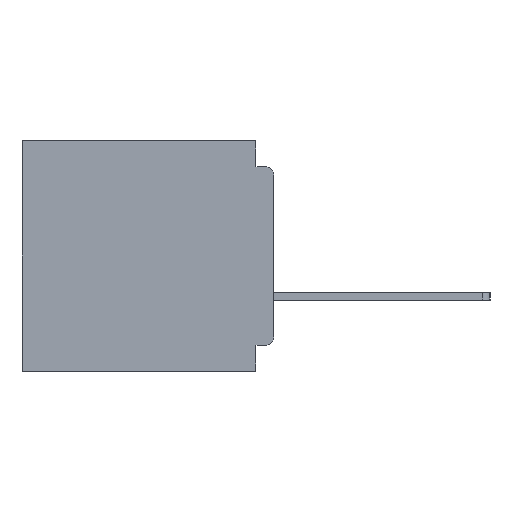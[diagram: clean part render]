
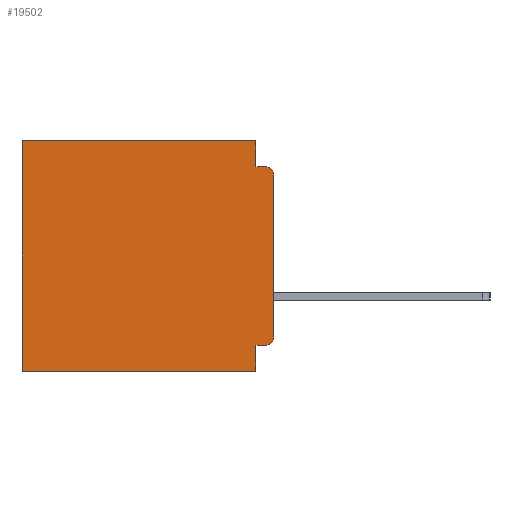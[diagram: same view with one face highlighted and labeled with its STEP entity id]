
A CAD part, left-side view. The second image highlights one B-rep face of the part: STEP entity #19502.
In plain terms, the highlighted planar face has unit normal (-1, 0, 0).
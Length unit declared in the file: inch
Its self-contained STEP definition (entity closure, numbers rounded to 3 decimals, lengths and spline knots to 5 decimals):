
#109 = CARTESIAN_POINT ( 'NONE',  ( 0.3, 0.015, -0.06 ) ) ;
#2106 = CARTESIAN_POINT ( 'NONE',  ( 0.3, 0.031, -0.4 ) ) ;
#2491 = EDGE_CURVE ( 'NONE', #35536, #6198, #42224, .T. ) ;
#3070 = LINE ( 'NONE', #46973, #23759 ) ;
#3792 = CIRCLE ( 'NONE', #16399, 0.015 ) ;
#3993 = CARTESIAN_POINT ( 'NONE',  ( 0.3, 0.437, -0.4 ) ) ;
#4067 = DIRECTION ( 'NONE',  ( 0., 0., -1. ) ) ;
#5150 = VECTOR ( 'NONE', #17080, 39.37008 ) ;
#5517 = CARTESIAN_POINT ( 'NONE',  ( 0.3, 0., -0.4 ) ) ;
#5836 = CARTESIAN_POINT ( 'NONE',  ( 0.3, 0.437, -0.4 ) ) ;
#6198 = VERTEX_POINT ( 'NONE', #5836 ) ;
#6887 = VERTEX_POINT ( 'NONE', #41497 ) ;
#7375 = VECTOR ( 'NONE', #49950, 39.37008 ) ;
#7682 = VECTOR ( 'NONE', #23790, 39.37008 ) ;
#9393 = ORIENTED_EDGE ( 'NONE', *, *, #21697, .F. ) ;
#9768 = ORIENTED_EDGE ( 'NONE', *, *, #14271, .F. ) ;
#10894 = VERTEX_POINT ( 'NONE', #34043 ) ;
#11126 = AXIS2_PLACEMENT_3D ( 'NONE', #14914, #41953, #18808 ) ;
#11199 = CARTESIAN_POINT ( 'NONE',  ( 0.3, 0.031, -0.355 ) ) ;
#11205 = CARTESIAN_POINT ( 'NONE',  ( 0.3, 0.031, 0. ) ) ;
#11536 = ORIENTED_EDGE ( 'NONE', *, *, #36013, .T. ) ;
#11788 = DIRECTION ( 'NONE',  ( 0., 0., -1. ) ) ;
#13599 = EDGE_CURVE ( 'NONE', #49246, #6198, #19241, .T. ) ;
#14271 = EDGE_CURVE ( 'NONE', #6887, #27284, #48869, .T. ) ;
#14914 = CARTESIAN_POINT ( 'NONE',  ( 0.3, 0.015, -0.34 ) ) ;
#15825 = CARTESIAN_POINT ( 'NONE',  ( 0.3, 0.031, -0.4 ) ) ;
#15903 = CARTESIAN_POINT ( 'NONE',  ( 0.3, 0.437, 0. ) ) ;
#16375 = DIRECTION ( 'NONE',  ( 1., 0., 0. ) ) ;
#16399 = AXIS2_PLACEMENT_3D ( 'NONE', #109, #27318, #4067 ) ;
#17080 = DIRECTION ( 'NONE',  ( 0., 0., -1. ) ) ;
#17122 = DIRECTION ( 'NONE',  ( 0., 1., 0. ) ) ;
#17203 = CARTESIAN_POINT ( 'NONE',  ( 0.3, 0.031, 0. ) ) ;
#18485 = FACE_OUTER_BOUND ( 'NONE', #36540, .T. ) ;
#18808 = DIRECTION ( 'NONE',  ( 0., 0., -1. ) ) ;
#18819 = ORIENTED_EDGE ( 'NONE', *, *, #21983, .T. ) ;
#19100 = EDGE_CURVE ( 'NONE', #24265, #35536, #31268, .T. ) ;
#19241 = LINE ( 'NONE', #3993, #38600 ) ;
#19502 = ADVANCED_FACE ( 'NONE', ( #18485 ), #31776, .F. ) ;
#19882 = CARTESIAN_POINT ( 'NONE',  ( 0.3, 0., -0.045 ) ) ;
#20841 = ORIENTED_EDGE ( 'NONE', *, *, #45400, .F. ) ;
#21107 = LINE ( 'NONE', #44178, #40495 ) ;
#21475 = DIRECTION ( 'NONE',  ( 0., 0., -1. ) ) ;
#21664 = VECTOR ( 'NONE', #45817, 39.37008 ) ;
#21697 = EDGE_CURVE ( 'NONE', #22167, #6887, #40722, .T. ) ;
#21983 = EDGE_CURVE ( 'NONE', #22167, #49246, #3070, .T. ) ;
#22167 = VERTEX_POINT ( 'NONE', #17203 ) ;
#23028 = EDGE_CURVE ( 'NONE', #31654, #27360, #27892, .T. ) ;
#23759 = VECTOR ( 'NONE', #31605, 39.37008 ) ;
#23790 = DIRECTION ( 'NONE',  ( 0., -1., 0. ) ) ;
#24265 = VERTEX_POINT ( 'NONE', #11199 ) ;
#25799 = CARTESIAN_POINT ( 'NONE',  ( 0.3, 0.015, -0.355 ) ) ;
#27284 = VERTEX_POINT ( 'NONE', #32142 ) ;
#27318 = DIRECTION ( 'NONE',  ( -1., 0., 0. ) ) ;
#27360 = VERTEX_POINT ( 'NONE', #36517 ) ;
#27892 = CIRCLE ( 'NONE', #11126, 0.015 ) ;
#27903 = CARTESIAN_POINT ( 'NONE',  ( 0.3, 0., -0.4 ) ) ;
#30729 = ORIENTED_EDGE ( 'NONE', *, *, #13599, .T. ) ;
#31268 = LINE ( 'NONE', #2106, #39122 ) ;
#31599 = ORIENTED_EDGE ( 'NONE', *, *, #2491, .F. ) ;
#31605 = DIRECTION ( 'NONE',  ( 0., 1., 0. ) ) ;
#31654 = VERTEX_POINT ( 'NONE', #25799 ) ;
#31776 = PLANE ( 'NONE',  #49595 ) ;
#32142 = CARTESIAN_POINT ( 'NONE',  ( 0.3, 0.015, -0.045 ) ) ;
#33873 = ORIENTED_EDGE ( 'NONE', *, *, #19100, .F. ) ;
#34043 = CARTESIAN_POINT ( 'NONE',  ( 0.3, 0., -0.06 ) ) ;
#34860 = ORIENTED_EDGE ( 'NONE', *, *, #43773, .F. ) ;
#35536 = VERTEX_POINT ( 'NONE', #15825 ) ;
#35546 = ORIENTED_EDGE ( 'NONE', *, *, #23028, .T. ) ;
#36013 = EDGE_CURVE ( 'NONE', #10894, #27284, #3792, .T. ) ;
#36517 = CARTESIAN_POINT ( 'NONE',  ( 0.3, 0., -0.34 ) ) ;
#36540 = EDGE_LOOP ( 'NONE', ( #20841, #11536, #9768, #9393, #18819, #30729, #31599, #33873, #34860, #35546 ) ) ;
#38600 = VECTOR ( 'NONE', #11788, 39.37008 ) ;
#39122 = VECTOR ( 'NONE', #21475, 39.37008 ) ;
#40495 = VECTOR ( 'NONE', #17122, 39.37008 ) ;
#40722 = LINE ( 'NONE', #11205, #7375 ) ;
#41497 = CARTESIAN_POINT ( 'NONE',  ( 0.3, 0.031, -0.045 ) ) ;
#41953 = DIRECTION ( 'NONE',  ( -1., 0., 0. ) ) ;
#42224 = LINE ( 'NONE', #45542, #21664 ) ;
#43441 = DIRECTION ( 'NONE',  ( 0., 0., -1. ) ) ;
#43773 = EDGE_CURVE ( 'NONE', #31654, #24265, #21107, .T. ) ;
#44178 = CARTESIAN_POINT ( 'NONE',  ( 0.3, 0., -0.355 ) ) ;
#45400 = EDGE_CURVE ( 'NONE', #10894, #27360, #47561, .T. ) ;
#45542 = CARTESIAN_POINT ( 'NONE',  ( 0.3, 0., -0.4 ) ) ;
#45817 = DIRECTION ( 'NONE',  ( 0., 1., 0. ) ) ;
#46973 = CARTESIAN_POINT ( 'NONE',  ( 0.3, 0., 0. ) ) ;
#47561 = LINE ( 'NONE', #5517, #5150 ) ;
#48869 = LINE ( 'NONE', #19882, #7682 ) ;
#49246 = VERTEX_POINT ( 'NONE', #15903 ) ;
#49595 = AXIS2_PLACEMENT_3D ( 'NONE', #27903, #16375, #43441 ) ;
#49950 = DIRECTION ( 'NONE',  ( 0., 0., -1. ) ) ;
